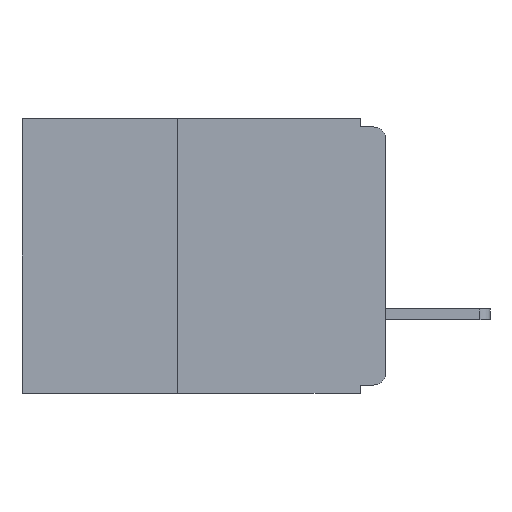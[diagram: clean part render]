
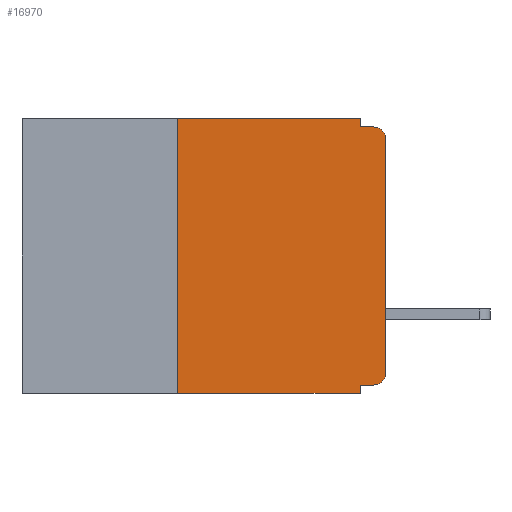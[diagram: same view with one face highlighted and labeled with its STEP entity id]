
A CAD part, left-side view. The second image highlights one B-rep face of the part: STEP entity #16970.
In plain terms, the highlighted planar face has unit normal (-1, 0, 0).
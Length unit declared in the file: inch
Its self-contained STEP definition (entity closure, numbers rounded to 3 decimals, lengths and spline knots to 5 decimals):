
#13 = DIRECTION ( 'NONE',  ( 0., 0., -1. ) ) ;
#226 = CARTESIAN_POINT ( 'NONE',  ( 0., 0.031, -0.33 ) ) ;
#254 = VERTEX_POINT ( 'NONE', #13372 ) ;
#412 = VERTEX_POINT ( 'NONE', #10186 ) ;
#885 = VERTEX_POINT ( 'NONE', #16489 ) ;
#1636 = ORIENTED_EDGE ( 'NONE', *, *, #25781, .F. ) ;
#2381 = LINE ( 'NONE', #18606, #23821 ) ;
#2721 = DIRECTION ( 'NONE',  ( -1., 0., 0. ) ) ;
#2773 = CARTESIAN_POINT ( 'NONE',  ( 0., 0., -0.01 ) ) ;
#3024 = CARTESIAN_POINT ( 'NONE',  ( 0., 0.031, -0.33 ) ) ;
#3410 = ORIENTED_EDGE ( 'NONE', *, *, #20930, .T. ) ;
#3524 = VECTOR ( 'NONE', #16140, 39.37008 ) ;
#4198 = LINE ( 'NONE', #26552, #3524 ) ;
#4810 = ORIENTED_EDGE ( 'NONE', *, *, #12347, .F. ) ;
#5056 = DIRECTION ( 'NONE',  ( 0., -1., 0. ) ) ;
#5275 = EDGE_CURVE ( 'NONE', #16992, #15782, #6804, .T. ) ;
#5325 = FACE_OUTER_BOUND ( 'NONE', #5807, .T. ) ;
#5807 = EDGE_LOOP ( 'NONE', ( #3410, #11069, #21832, #4810, #10606, #8555, #23455, #10777, #1636, #20639 ) ) ;
#6804 = CIRCLE ( 'NONE', #24164, 0.015 ) ;
#7903 = EDGE_CURVE ( 'NONE', #885, #27349, #10133, .T. ) ;
#8111 = VECTOR ( 'NONE', #5056, 39.37008 ) ;
#8169 = VECTOR ( 'NONE', #19560, 39.37008 ) ;
#8464 = AXIS2_PLACEMENT_3D ( 'NONE', #23640, #10910, #25750 ) ;
#8476 = VECTOR ( 'NONE', #19408, 39.37008 ) ;
#8555 = ORIENTED_EDGE ( 'NONE', *, *, #21991, .F. ) ;
#8727 = CARTESIAN_POINT ( 'NONE',  ( 0., 0.015, -0.01 ) ) ;
#8796 = CARTESIAN_POINT ( 'NONE',  ( 0., 0.015, -0.32 ) ) ;
#9854 = DIRECTION ( 'NONE',  ( 0., 1., 0. ) ) ;
#10133 = CIRCLE ( 'NONE', #23681, 0.015 ) ;
#10186 = CARTESIAN_POINT ( 'NONE',  ( 0., 0.25, -0.33 ) ) ;
#10606 = ORIENTED_EDGE ( 'NONE', *, *, #22432, .F. ) ;
#10722 = CARTESIAN_POINT ( 'NONE',  ( 0., 0.437, 0. ) ) ;
#10777 = ORIENTED_EDGE ( 'NONE', *, *, #24836, .F. ) ;
#10910 = DIRECTION ( 'NONE',  ( 1., 0., 0. ) ) ;
#11021 = VERTEX_POINT ( 'NONE', #23707 ) ;
#11069 = ORIENTED_EDGE ( 'NONE', *, *, #7903, .T. ) ;
#11410 = CARTESIAN_POINT ( 'NONE',  ( 0., 0.25, -0.33 ) ) ;
#12347 = EDGE_CURVE ( 'NONE', #27121, #15594, #15084, .T. ) ;
#12388 = EDGE_CURVE ( 'NONE', #412, #15129, #4198, .T. ) ;
#13038 = DIRECTION ( 'NONE',  ( -1., 0., 0. ) ) ;
#13372 = CARTESIAN_POINT ( 'NONE',  ( 0., 0.031, -0.32 ) ) ;
#13589 = VECTOR ( 'NONE', #19339, 39.37008 ) ;
#13625 = DIRECTION ( 'NONE',  ( 0., 0., 1. ) ) ;
#13885 = CARTESIAN_POINT ( 'NONE',  ( 0., 0.031, 0. ) ) ;
#14404 = EDGE_CURVE ( 'NONE', #15594, #27349, #25142, .T. ) ;
#14667 = LINE ( 'NONE', #226, #8169 ) ;
#15084 = LINE ( 'NONE', #13885, #25581 ) ;
#15124 = PLANE ( 'NONE',  #8464 ) ;
#15129 = VERTEX_POINT ( 'NONE', #3024 ) ;
#15594 = VERTEX_POINT ( 'NONE', #23776 ) ;
#15732 = CARTESIAN_POINT ( 'NONE',  ( 0., 0.015, -0.025 ) ) ;
#15782 = VERTEX_POINT ( 'NONE', #19588 ) ;
#16140 = DIRECTION ( 'NONE',  ( 0., -1., 0. ) ) ;
#16489 = CARTESIAN_POINT ( 'NONE',  ( 0., 0., -0.025 ) ) ;
#16970 = ADVANCED_FACE ( 'NONE', ( #5325 ), #15124, .F. ) ;
#16992 = VERTEX_POINT ( 'NONE', #8796 ) ;
#17835 = DIRECTION ( 'NONE',  ( 0., 0., -1. ) ) ;
#18606 = CARTESIAN_POINT ( 'NONE',  ( 0., 0., -0.32 ) ) ;
#19339 = DIRECTION ( 'NONE',  ( 0., -1., 0. ) ) ;
#19408 = DIRECTION ( 'NONE',  ( 0., 0., 1. ) ) ;
#19560 = DIRECTION ( 'NONE',  ( 0., 0., -1. ) ) ;
#19588 = CARTESIAN_POINT ( 'NONE',  ( 0., 0., -0.305 ) ) ;
#19917 = LINE ( 'NONE', #23531, #8476 ) ;
#20191 = VECTOR ( 'NONE', #13625, 39.37008 ) ;
#20639 = ORIENTED_EDGE ( 'NONE', *, *, #5275, .T. ) ;
#20844 = LINE ( 'NONE', #11410, #20191 ) ;
#20930 = EDGE_CURVE ( 'NONE', #15782, #885, #19917, .T. ) ;
#20936 = CARTESIAN_POINT ( 'NONE',  ( 0., 0.031, 0. ) ) ;
#21832 = ORIENTED_EDGE ( 'NONE', *, *, #14404, .F. ) ;
#21991 = EDGE_CURVE ( 'NONE', #412, #11021, #20844, .T. ) ;
#22432 = EDGE_CURVE ( 'NONE', #11021, #27121, #25447, .T. ) ;
#23455 = ORIENTED_EDGE ( 'NONE', *, *, #12388, .T. ) ;
#23531 = CARTESIAN_POINT ( 'NONE',  ( 0., 0., 0. ) ) ;
#23640 = CARTESIAN_POINT ( 'NONE',  ( 0., 0.437, 0. ) ) ;
#23681 = AXIS2_PLACEMENT_3D ( 'NONE', #15732, #2721, #17835 ) ;
#23707 = CARTESIAN_POINT ( 'NONE',  ( 0., 0.25, 0. ) ) ;
#23776 = CARTESIAN_POINT ( 'NONE',  ( 0., 0.031, -0.01 ) ) ;
#23821 = VECTOR ( 'NONE', #9854, 39.37008 ) ;
#24164 = AXIS2_PLACEMENT_3D ( 'NONE', #25675, #13038, #13 ) ;
#24836 = EDGE_CURVE ( 'NONE', #254, #15129, #14667, .T. ) ;
#25142 = LINE ( 'NONE', #2773, #8111 ) ;
#25447 = LINE ( 'NONE', #10722, #13589 ) ;
#25581 = VECTOR ( 'NONE', #26460, 39.37008 ) ;
#25675 = CARTESIAN_POINT ( 'NONE',  ( 0., 0.015, -0.305 ) ) ;
#25750 = DIRECTION ( 'NONE',  ( 0., 0., -1. ) ) ;
#25781 = EDGE_CURVE ( 'NONE', #16992, #254, #2381, .T. ) ;
#26460 = DIRECTION ( 'NONE',  ( 0., 0., -1. ) ) ;
#26552 = CARTESIAN_POINT ( 'NONE',  ( 0., 0.437, -0.33 ) ) ;
#27121 = VERTEX_POINT ( 'NONE', #20936 ) ;
#27349 = VERTEX_POINT ( 'NONE', #8727 ) ;
